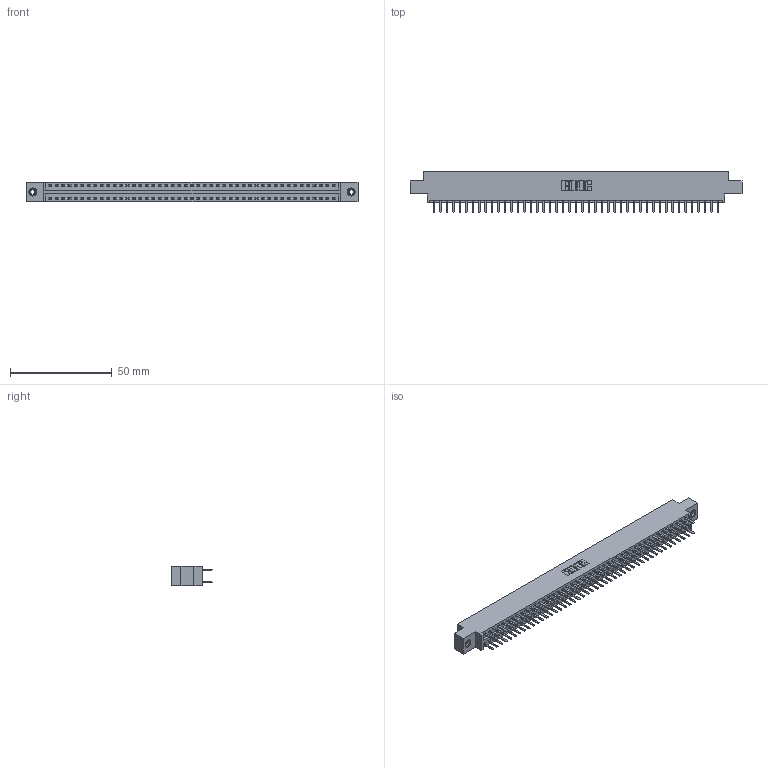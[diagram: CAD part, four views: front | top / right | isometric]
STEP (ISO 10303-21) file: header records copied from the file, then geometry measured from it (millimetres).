
FILE_DESCRIPTION (( 'STEP AP203' ), '1' );
FILE_NAME ('396-090-520-808.STEP', '2018-09-12T04:19:57', ( '' ), ( '' ), 'SwSTEP 2.0', 'SolidWorks 2016', '' );
FILE_SCHEMA (( 'CONFIG_CONTROL_DESIGN' ));
Length unit declared in the file: inch
Products named in the file (4): 396-090-520-808; 346 Part_0.170 Offset - 0.156 Dia-TI; 345-292-001_345-293-120; 345-250-001_345-250-003-102
Assembly tree (93 placements, depth 2):
  396-090-520-808
    346 Part_0.170 Offset - 0.156 Dia-TI
    345-292-001_345-293-120  x90
    345-250-001_345-250-003-102  x2
Bounding box: 163.45 x 20.02 x 9.4 mm (x, y, z)
Volume: 15760.9 mm3; surface area: 21818.5 mm2
Topology: 93 solids, 93 shells, 5226 faces, 15147 edges, 9850 vertices
Faces by surface type: plane 3442, cylinder 1768, cone 12, torus 4
Entity records: 30396 total; most frequent: CARTESIAN_POINT 5003, ORIENTED_EDGE 4918, DIRECTION 4473, EDGE_CURVE 2459, VECTOR 2123, LINE 2123, VERTEX_POINT 1632, AXIS2_PLACEMENT_3D 1175
